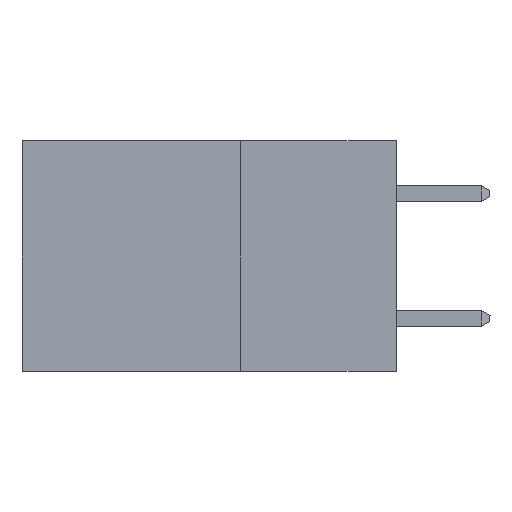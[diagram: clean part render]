
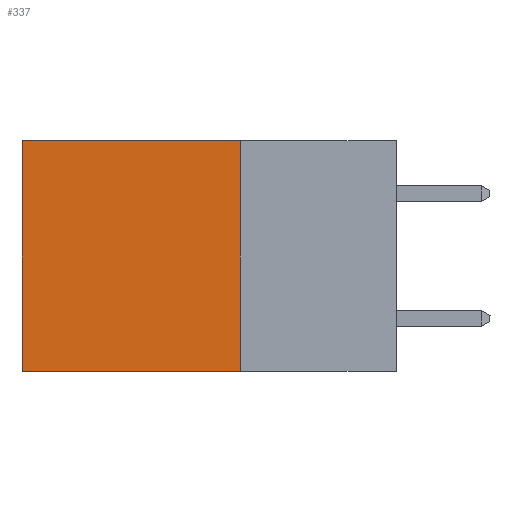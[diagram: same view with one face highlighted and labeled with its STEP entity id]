
A CAD part, left-side view. The second image highlights one B-rep face of the part: STEP entity #337.
In plain terms, the highlighted planar face has unit normal (-1, 0, 0).
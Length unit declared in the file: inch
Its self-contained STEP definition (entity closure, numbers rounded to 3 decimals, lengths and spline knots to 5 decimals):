
#337 = ADVANCED_FACE ( 'NONE', ( #619 ), #18999, .F. ) ;
#365 = EDGE_CURVE ( 'NONE', #11808, #2375, #9608, .T. ) ;
#619 = FACE_OUTER_BOUND ( 'NONE', #8408, .T. ) ;
#1021 = DIRECTION ( 'NONE',  ( 1., 0., 0. ) ) ;
#1087 = VECTOR ( 'NONE', #13151, 39.37008 ) ;
#1743 = CARTESIAN_POINT ( 'NONE',  ( 0.2615, 0.6, -0.37 ) ) ;
#2375 = VERTEX_POINT ( 'NONE', #23175 ) ;
#3954 = VERTEX_POINT ( 'NONE', #13224 ) ;
#4257 = VECTOR ( 'NONE', #24292, 39.37008 ) ;
#4472 = VECTOR ( 'NONE', #22861, 39.37008 ) ;
#5263 = ORIENTED_EDGE ( 'NONE', *, *, #13625, .T. ) ;
#5387 = ORIENTED_EDGE ( 'NONE', *, *, #6554, .F. ) ;
#6554 = EDGE_CURVE ( 'NONE', #2375, #15260, #19448, .T. ) ;
#8008 = VECTOR ( 'NONE', #17359, 39.37008 ) ;
#8408 = EDGE_LOOP ( 'NONE', ( #16817, #5387, #13566, #5263 ) ) ;
#9257 = CARTESIAN_POINT ( 'NONE',  ( 0.2615, 0.25, -0.37 ) ) ;
#9608 = LINE ( 'NONE', #19106, #4472 ) ;
#9701 = CARTESIAN_POINT ( 'NONE',  ( 0.2615, 0.6, -0.37 ) ) ;
#11287 = CARTESIAN_POINT ( 'NONE',  ( 0.2615, 0.25, 0. ) ) ;
#11808 = VERTEX_POINT ( 'NONE', #24309 ) ;
#13109 = EDGE_CURVE ( 'NONE', #3954, #15260, #18128, .T. ) ;
#13151 = DIRECTION ( 'NONE',  ( 0., 1., 0. ) ) ;
#13224 = CARTESIAN_POINT ( 'NONE',  ( 0.2615, 0.6, 0. ) ) ;
#13566 = ORIENTED_EDGE ( 'NONE', *, *, #365, .F. ) ;
#13625 = EDGE_CURVE ( 'NONE', #11808, #3954, #21302, .T. ) ;
#15260 = VERTEX_POINT ( 'NONE', #1743 ) ;
#16817 = ORIENTED_EDGE ( 'NONE', *, *, #13109, .T. ) ;
#17359 = DIRECTION ( 'NONE',  ( 0., 0., -1. ) ) ;
#18128 = LINE ( 'NONE', #9701, #8008 ) ;
#18999 = PLANE ( 'NONE',  #21649 ) ;
#19106 = CARTESIAN_POINT ( 'NONE',  ( 0.2615, 0.25, -0.37 ) ) ;
#19448 = LINE ( 'NONE', #9257, #4257 ) ;
#20253 = DIRECTION ( 'NONE',  ( 0., 0., -1. ) ) ;
#21302 = LINE ( 'NONE', #11287, #1087 ) ;
#21649 = AXIS2_PLACEMENT_3D ( 'NONE', #23975, #1021, #20253 ) ;
#22861 = DIRECTION ( 'NONE',  ( 0., 0., -1. ) ) ;
#23175 = CARTESIAN_POINT ( 'NONE',  ( 0.2615, 0.25, -0.37 ) ) ;
#23975 = CARTESIAN_POINT ( 'NONE',  ( 0.2615, 0.25, -0.37 ) ) ;
#24292 = DIRECTION ( 'NONE',  ( 0., 1., 0. ) ) ;
#24309 = CARTESIAN_POINT ( 'NONE',  ( 0.2615, 0.25, 0. ) ) ;
